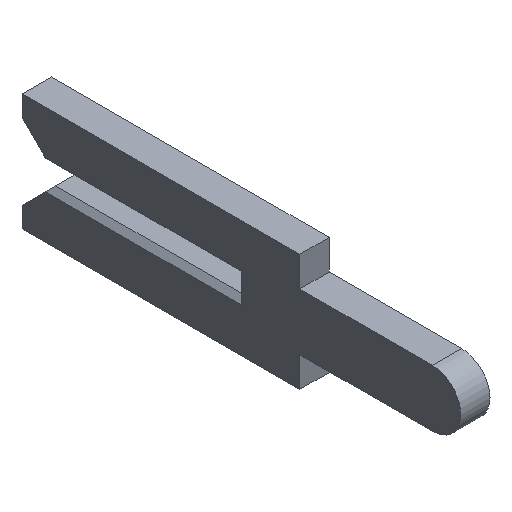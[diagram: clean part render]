
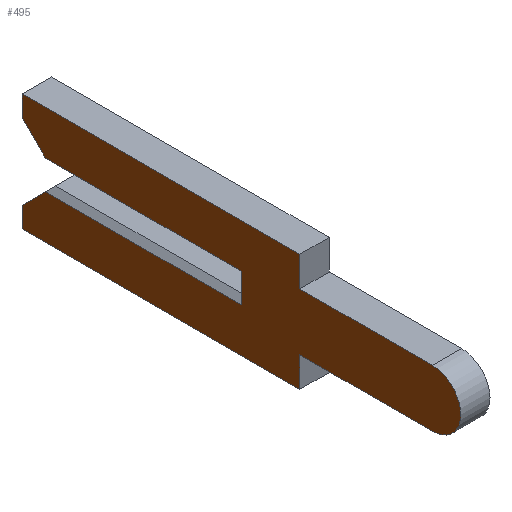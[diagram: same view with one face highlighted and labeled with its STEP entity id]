
A CAD part, isometric view. The second image highlights one B-rep face of the part: STEP entity #495.
In plain terms, the highlighted planar face has unit normal (-1, 0, 0).
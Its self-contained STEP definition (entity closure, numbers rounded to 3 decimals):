
#8 = EDGE_CURVE ( 'NONE', #517, #261, #66, .T. ) ;
#15 = ORIENTED_EDGE ( 'NONE', *, *, #522, .F. ) ;
#31 = CARTESIAN_POINT ( 'NONE',  ( -0.254, 0., -0.254 ) ) ;
#32 = EDGE_CURVE ( 'NONE', #295, #517, #412, .T. ) ;
#35 = CARTESIAN_POINT ( 'NONE',  ( -0.254, -1.016, 1.016 ) ) ;
#42 = VERTEX_POINT ( 'NONE', #100 ) ;
#52 = VECTOR ( 'NONE', #814, 1000. ) ;
#59 = LINE ( 'NONE', #438, #282 ) ;
#61 = LINE ( 'NONE', #597, #393 ) ;
#63 = AXIS2_PLACEMENT_3D ( 'NONE', #612, #408, #474 ) ;
#66 = LINE ( 'NONE', #337, #255 ) ;
#71 = VECTOR ( 'NONE', #152, 1000. ) ;
#73 = CARTESIAN_POINT ( 'NONE',  ( -0.254, 0., 0.254 ) ) ;
#80 = LINE ( 'NONE', #493, #745 ) ;
#84 = CARTESIAN_POINT ( 'NONE',  ( -0.254, -1.016, -0.495 ) ) ;
#93 = VERTEX_POINT ( 'NONE', #84 ) ;
#98 = EDGE_CURVE ( 'NONE', #118, #342, #619, .T. ) ;
#100 = CARTESIAN_POINT ( 'NONE',  ( -0.254, 3.81, 0.66 ) ) ;
#102 = VERTEX_POINT ( 'NONE', #162 ) ;
#118 = VERTEX_POINT ( 'NONE', #313 ) ;
#123 = ORIENTED_EDGE ( 'NONE', *, *, #8, .F. ) ;
#126 = DIRECTION ( 'NONE',  ( 0., 1., 0. ) ) ;
#144 = ORIENTED_EDGE ( 'NONE', *, *, #779, .F. ) ;
#148 = ORIENTED_EDGE ( 'NONE', *, *, #706, .F. ) ;
#152 = DIRECTION ( 'NONE',  ( 0., 0.707, 0.707 ) ) ;
#162 = CARTESIAN_POINT ( 'NONE',  ( -0.254, 3.404, -0.254 ) ) ;
#166 = EDGE_CURVE ( 'NONE', #261, #118, #581, .T. ) ;
#169 = CARTESIAN_POINT ( 'NONE',  ( -0.254, 3.315, -0.165 ) ) ;
#177 = DIRECTION ( 'NONE',  ( 0., -1., 0. ) ) ;
#193 = LINE ( 'NONE', #740, #52 ) ;
#210 = LINE ( 'NONE', #276, #528 ) ;
#217 = ORIENTED_EDGE ( 'NONE', *, *, #675, .T. ) ;
#223 = DIRECTION ( 'NONE',  ( 1., 0., 0. ) ) ;
#229 = LINE ( 'NONE', #550, #257 ) ;
#231 = VECTOR ( 'NONE', #677, 1000. ) ;
#255 = VECTOR ( 'NONE', #543, 1000. ) ;
#257 = VECTOR ( 'NONE', #350, 1000. ) ;
#260 = CARTESIAN_POINT ( 'NONE',  ( -0.254, 3.81, 1.016 ) ) ;
#261 = VERTEX_POINT ( 'NONE', #270 ) ;
#266 = VECTOR ( 'NONE', #552, 1000. ) ;
#270 = CARTESIAN_POINT ( 'NONE',  ( -0.254, -1.016, 0.495 ) ) ;
#273 = CARTESIAN_POINT ( 'NONE',  ( -0.254, 3.315, 0.165 ) ) ;
#276 = CARTESIAN_POINT ( 'NONE',  ( -0.254, 3.81, 0.66 ) ) ;
#282 = VECTOR ( 'NONE', #126, 1000. ) ;
#295 = VERTEX_POINT ( 'NONE', #260 ) ;
#313 = CARTESIAN_POINT ( 'NONE',  ( -0.254, -3.315, 0.495 ) ) ;
#317 = ORIENTED_EDGE ( 'NONE', *, *, #32, .F. ) ;
#325 = EDGE_CURVE ( 'NONE', #342, #93, #737, .T. ) ;
#326 = ORIENTED_EDGE ( 'NONE', *, *, #661, .F. ) ;
#328 = LINE ( 'NONE', #273, #71 ) ;
#334 = CARTESIAN_POINT ( 'NONE',  ( -0.254, -3.315, 0. ) ) ;
#337 = CARTESIAN_POINT ( 'NONE',  ( -0.254, -1.016, 1.016 ) ) ;
#338 = DIRECTION ( 'NONE',  ( 0., 0., -1. ) ) ;
#342 = VERTEX_POINT ( 'NONE', #406 ) ;
#345 = DIRECTION ( 'NONE',  ( 0., 0., -1. ) ) ;
#350 = DIRECTION ( 'NONE',  ( 0., -1., 0. ) ) ;
#355 = VERTEX_POINT ( 'NONE', #724 ) ;
#384 = EDGE_CURVE ( 'NONE', #42, #295, #210, .T. ) ;
#391 = ORIENTED_EDGE ( 'NONE', *, *, #566, .F. ) ;
#393 = VECTOR ( 'NONE', #338, 1000. ) ;
#394 = DIRECTION ( 'NONE',  ( 0., 1., 0. ) ) ;
#396 = CARTESIAN_POINT ( 'NONE',  ( -0.254, -1.016, -0.495 ) ) ;
#401 = CARTESIAN_POINT ( 'NONE',  ( -0.254, -1.016, -1.016 ) ) ;
#402 = VECTOR ( 'NONE', #577, 1000. ) ;
#405 = CARTESIAN_POINT ( 'NONE',  ( -0.254, 3.404, 0.254 ) ) ;
#406 = CARTESIAN_POINT ( 'NONE',  ( -0.254, -3.315, -0.495 ) ) ;
#408 = DIRECTION ( 'NONE',  ( 1., 0., 0. ) ) ;
#411 = EDGE_CURVE ( 'NONE', #93, #416, #61, .T. ) ;
#412 = LINE ( 'NONE', #541, #266 ) ;
#416 = VERTEX_POINT ( 'NONE', #401 ) ;
#418 = ORIENTED_EDGE ( 'NONE', *, *, #98, .F. ) ;
#438 = CARTESIAN_POINT ( 'NONE',  ( -0.254, 3.81, -1.016 ) ) ;
#443 = VERTEX_POINT ( 'NONE', #31 ) ;
#444 = VERTEX_POINT ( 'NONE', #544 ) ;
#459 = VERTEX_POINT ( 'NONE', #405 ) ;
#474 = DIRECTION ( 'NONE',  ( 0., 0., -1. ) ) ;
#485 = ORIENTED_EDGE ( 'NONE', *, *, #325, .F. ) ;
#489 = EDGE_LOOP ( 'NONE', ( #217, #326, #148, #391, #632, #144, #536, #485, #418, #651, #123, #317, #687, #15 ) ) ;
#492 = VECTOR ( 'NONE', #394, 1000. ) ;
#493 = CARTESIAN_POINT ( 'NONE',  ( -0.254, 3.81, -0.66 ) ) ;
#495 = ADVANCED_FACE ( 'NONE', ( #824 ), #539, .F. ) ;
#517 = VERTEX_POINT ( 'NONE', #35 ) ;
#522 = EDGE_CURVE ( 'NONE', #459, #42, #328, .T. ) ;
#524 = VERTEX_POINT ( 'NONE', #73 ) ;
#528 = VECTOR ( 'NONE', #530, 1000. ) ;
#530 = DIRECTION ( 'NONE',  ( 0., 0., 1. ) ) ;
#536 = ORIENTED_EDGE ( 'NONE', *, *, #411, .F. ) ;
#539 = PLANE ( 'NONE',  #766 ) ;
#541 = CARTESIAN_POINT ( 'NONE',  ( -0.254, 3.81, 1.016 ) ) ;
#543 = DIRECTION ( 'NONE',  ( 0., 0., -1. ) ) ;
#544 = CARTESIAN_POINT ( 'NONE',  ( -0.254, 3.81, -1.016 ) ) ;
#550 = CARTESIAN_POINT ( 'NONE',  ( -0.254, 3.81, 0.254 ) ) ;
#552 = DIRECTION ( 'NONE',  ( 0., -1., 0. ) ) ;
#553 = LINE ( 'NONE', #169, #231 ) ;
#560 = CARTESIAN_POINT ( 'NONE',  ( -0.254, -3.315, -0.254 ) ) ;
#566 = EDGE_CURVE ( 'NONE', #355, #102, #553, .T. ) ;
#577 = DIRECTION ( 'NONE',  ( 0., -1., 0. ) ) ;
#581 = LINE ( 'NONE', #701, #402 ) ;
#597 = CARTESIAN_POINT ( 'NONE',  ( -0.254, -1.016, -1.016 ) ) ;
#612 = CARTESIAN_POINT ( 'NONE',  ( -0.254, -3.315, 0. ) ) ;
#619 = CIRCLE ( 'NONE', #63, 0.495 ) ;
#632 = ORIENTED_EDGE ( 'NONE', *, *, #637, .F. ) ;
#637 = EDGE_CURVE ( 'NONE', #444, #355, #80, .T. ) ;
#651 = ORIENTED_EDGE ( 'NONE', *, *, #166, .F. ) ;
#661 = EDGE_CURVE ( 'NONE', #443, #524, #193, .T. ) ;
#671 = VECTOR ( 'NONE', #177, 1000. ) ;
#675 = EDGE_CURVE ( 'NONE', #459, #524, #229, .T. ) ;
#677 = DIRECTION ( 'NONE',  ( 0., -0.707, 0.707 ) ) ;
#687 = ORIENTED_EDGE ( 'NONE', *, *, #384, .F. ) ;
#701 = CARTESIAN_POINT ( 'NONE',  ( -0.254, -1.016, 0.495 ) ) ;
#706 = EDGE_CURVE ( 'NONE', #102, #443, #801, .T. ) ;
#724 = CARTESIAN_POINT ( 'NONE',  ( -0.254, 3.81, -0.66 ) ) ;
#737 = LINE ( 'NONE', #396, #492 ) ;
#740 = CARTESIAN_POINT ( 'NONE',  ( -0.254, 0., 0.165 ) ) ;
#745 = VECTOR ( 'NONE', #818, 1000. ) ;
#766 = AXIS2_PLACEMENT_3D ( 'NONE', #334, #223, #345 ) ;
#779 = EDGE_CURVE ( 'NONE', #416, #444, #59, .T. ) ;
#801 = LINE ( 'NONE', #560, #671 ) ;
#814 = DIRECTION ( 'NONE',  ( 0., 0., 1. ) ) ;
#818 = DIRECTION ( 'NONE',  ( 0., 0., 1. ) ) ;
#824 = FACE_OUTER_BOUND ( 'NONE', #489, .T. ) ;
